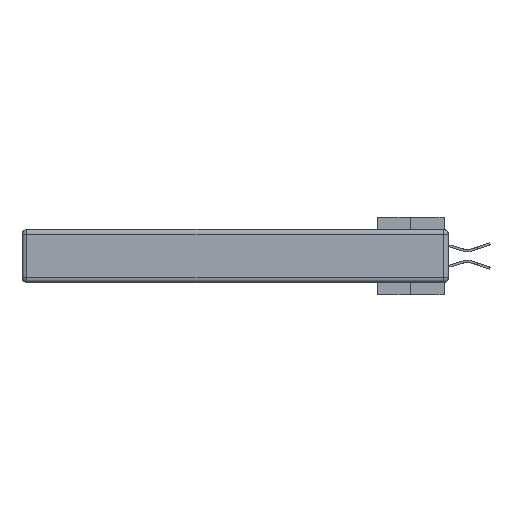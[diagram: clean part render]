
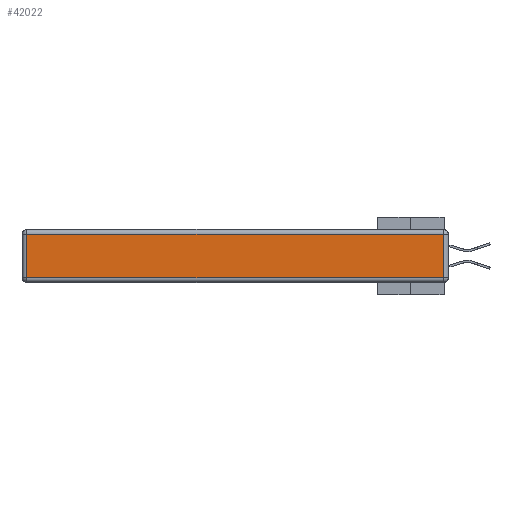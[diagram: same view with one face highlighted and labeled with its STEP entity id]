
A CAD part, left-side view. The second image highlights one B-rep face of the part: STEP entity #42022.
In plain terms, the highlighted planar face has unit normal (-1, 0, 0).
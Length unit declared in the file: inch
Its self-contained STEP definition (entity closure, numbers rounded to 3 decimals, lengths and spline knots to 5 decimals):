
#1215 = VERTEX_POINT ( 'NONE', #11675 ) ;
#2460 = CARTESIAN_POINT ( 'NONE',  ( 0., 0.03, -0.03 ) ) ;
#2927 = LINE ( 'NONE', #26455, #23633 ) ;
#3064 = DIRECTION ( 'NONE',  ( 0., 1., 0. ) ) ;
#3081 = DIRECTION ( 'NONE',  ( -1., 0., 0. ) ) ;
#3337 = LINE ( 'NONE', #23557, #33279 ) ;
#4468 = VECTOR ( 'NONE', #3064, 39.37008 ) ;
#5631 = EDGE_CURVE ( 'NONE', #31787, #31968, #2927, .T. ) ;
#5771 = DIRECTION ( 'NONE',  ( 0., 0., 1. ) ) ;
#6317 = LINE ( 'NONE', #9608, #32976 ) ;
#7711 = EDGE_CURVE ( 'NONE', #31968, #1215, #37114, .T. ) ;
#9406 = DIRECTION ( 'NONE',  ( 0., 0., 1. ) ) ;
#9608 = CARTESIAN_POINT ( 'NONE',  ( 0., 0., -0.313 ) ) ;
#11675 = CARTESIAN_POINT ( 'NONE',  ( 0., 2.72, -0.03 ) ) ;
#13400 = DIRECTION ( 'NONE',  ( 0., -1., 0. ) ) ;
#13870 = ORIENTED_EDGE ( 'NONE', *, *, #32293, .T. ) ;
#15116 = ORIENTED_EDGE ( 'NONE', *, *, #7711, .T. ) ;
#15773 = EDGE_LOOP ( 'NONE', ( #13870, #16042, #15116, #32856 ) ) ;
#16042 = ORIENTED_EDGE ( 'NONE', *, *, #5631, .T. ) ;
#17844 = CARTESIAN_POINT ( 'NONE',  ( 0., 0.03, -0.313 ) ) ;
#20353 = DIRECTION ( 'NONE',  ( 0., 0., -1. ) ) ;
#20727 = CARTESIAN_POINT ( 'NONE',  ( 0., 2.75, -0.03 ) ) ;
#21597 = FACE_OUTER_BOUND ( 'NONE', #15773, .T. ) ;
#21778 = AXIS2_PLACEMENT_3D ( 'NONE', #40630, #3081, #9406 ) ;
#23557 = CARTESIAN_POINT ( 'NONE',  ( 0., 2.72, -0.343 ) ) ;
#23633 = VECTOR ( 'NONE', #5771, 39.37008 ) ;
#26455 = CARTESIAN_POINT ( 'NONE',  ( 0., 0.03, -0.343 ) ) ;
#26975 = PLANE ( 'NONE',  #21778 ) ;
#28195 = VERTEX_POINT ( 'NONE', #36521 ) ;
#31787 = VERTEX_POINT ( 'NONE', #17844 ) ;
#31968 = VERTEX_POINT ( 'NONE', #2460 ) ;
#32293 = EDGE_CURVE ( 'NONE', #28195, #31787, #6317, .T. ) ;
#32856 = ORIENTED_EDGE ( 'NONE', *, *, #44934, .T. ) ;
#32976 = VECTOR ( 'NONE', #13400, 39.37008 ) ;
#33279 = VECTOR ( 'NONE', #20353, 39.37008 ) ;
#36521 = CARTESIAN_POINT ( 'NONE',  ( 0., 2.72, -0.313 ) ) ;
#37114 = LINE ( 'NONE', #20727, #4468 ) ;
#40630 = CARTESIAN_POINT ( 'NONE',  ( 0., 0., -0.343 ) ) ;
#42022 = ADVANCED_FACE ( 'NONE', ( #21597 ), #26975, .T. ) ;
#44934 = EDGE_CURVE ( 'NONE', #1215, #28195, #3337, .T. ) ;
